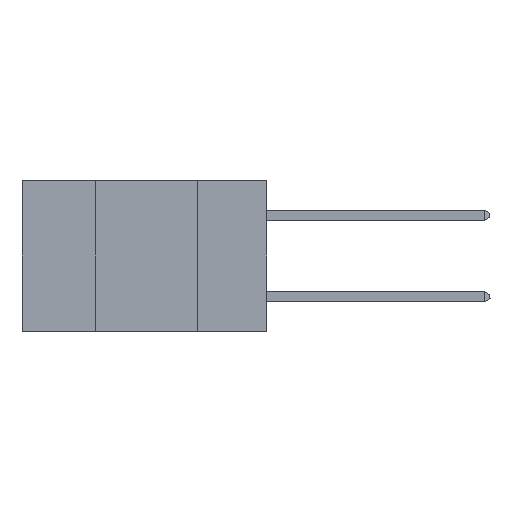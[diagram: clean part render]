
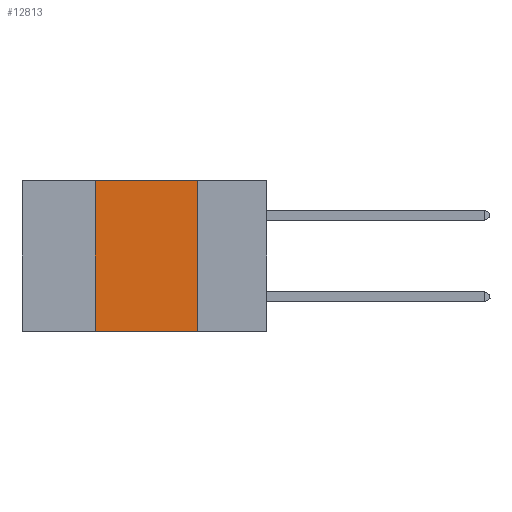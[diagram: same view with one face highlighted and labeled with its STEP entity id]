
A CAD part, left-side view. The second image highlights one B-rep face of the part: STEP entity #12813.
In plain terms, the highlighted planar face has unit normal (-1, 0, 0).
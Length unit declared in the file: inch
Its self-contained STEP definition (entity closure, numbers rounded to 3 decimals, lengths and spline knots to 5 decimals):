
#699 = DIRECTION ( 'NONE',  ( 0., -1., 0. ) ) ;
#1058 = EDGE_CURVE ( 'NONE', #10843, #15031, #15472, .T. ) ;
#1161 = DIRECTION ( 'NONE',  ( 0., 0., 1. ) ) ;
#1506 = EDGE_CURVE ( 'NONE', #2836, #10843, #19618, .T. ) ;
#2087 = DIRECTION ( 'NONE',  ( 1., 0., 0. ) ) ;
#2669 = VECTOR ( 'NONE', #2930, 39.37008 ) ;
#2836 = VERTEX_POINT ( 'NONE', #10239 ) ;
#2930 = DIRECTION ( 'NONE',  ( 0., 0., -1. ) ) ;
#2953 = EDGE_CURVE ( 'NONE', #6359, #15031, #19805, .T. ) ;
#3652 = CARTESIAN_POINT ( 'NONE',  ( 0., 0.6, 0. ) ) ;
#3819 = ORIENTED_EDGE ( 'NONE', *, *, #1506, .F. ) ;
#4129 = DIRECTION ( 'NONE',  ( 0., -1., 0. ) ) ;
#4282 = LINE ( 'NONE', #9110, #16500 ) ;
#4572 = CARTESIAN_POINT ( 'NONE',  ( 0., 0.17, 0. ) ) ;
#5183 = ORIENTED_EDGE ( 'NONE', *, *, #1058, .F. ) ;
#6359 = VERTEX_POINT ( 'NONE', #8405 ) ;
#7171 = CARTESIAN_POINT ( 'NONE',  ( 0., 0.6, 0. ) ) ;
#8405 = CARTESIAN_POINT ( 'NONE',  ( 0., 0.42, -0.37 ) ) ;
#9006 = EDGE_CURVE ( 'NONE', #6359, #2836, #4282, .T. ) ;
#9110 = CARTESIAN_POINT ( 'NONE',  ( 0., 0.42, 0. ) ) ;
#9440 = ORIENTED_EDGE ( 'NONE', *, *, #9006, .F. ) ;
#10239 = CARTESIAN_POINT ( 'NONE',  ( 0., 0.42, 0. ) ) ;
#10843 = VERTEX_POINT ( 'NONE', #14519 ) ;
#11731 = PLANE ( 'NONE',  #12755 ) ;
#12413 = ORIENTED_EDGE ( 'NONE', *, *, #2953, .T. ) ;
#12755 = AXIS2_PLACEMENT_3D ( 'NONE', #3652, #2087, #13325 ) ;
#12813 = ADVANCED_FACE ( 'NONE', ( #17580 ), #11731, .F. ) ;
#13189 = EDGE_LOOP ( 'NONE', ( #5183, #3819, #9440, #12413 ) ) ;
#13325 = DIRECTION ( 'NONE',  ( 0., 0., -1. ) ) ;
#14519 = CARTESIAN_POINT ( 'NONE',  ( 0., 0.17, 0. ) ) ;
#15031 = VERTEX_POINT ( 'NONE', #17637 ) ;
#15154 = VECTOR ( 'NONE', #4129, 39.37008 ) ;
#15451 = VECTOR ( 'NONE', #699, 39.37008 ) ;
#15472 = LINE ( 'NONE', #4572, #2669 ) ;
#16500 = VECTOR ( 'NONE', #1161, 39.37008 ) ;
#17580 = FACE_OUTER_BOUND ( 'NONE', #13189, .T. ) ;
#17637 = CARTESIAN_POINT ( 'NONE',  ( 0., 0.17, -0.37 ) ) ;
#18443 = CARTESIAN_POINT ( 'NONE',  ( 0., 0.6, -0.37 ) ) ;
#19618 = LINE ( 'NONE', #7171, #15451 ) ;
#19805 = LINE ( 'NONE', #18443, #15154 ) ;
